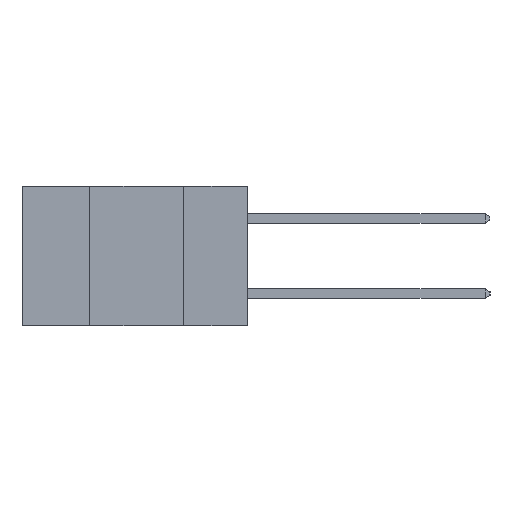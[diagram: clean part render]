
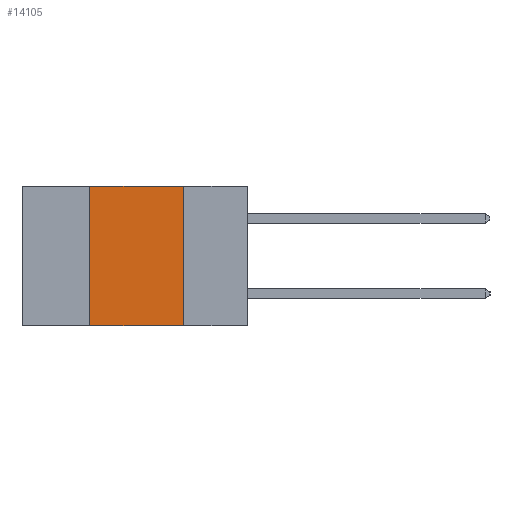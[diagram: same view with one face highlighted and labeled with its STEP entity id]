
A CAD part, left-side view. The second image highlights one B-rep face of the part: STEP entity #14105.
In plain terms, the highlighted planar face has unit normal (-1, 0, 0).
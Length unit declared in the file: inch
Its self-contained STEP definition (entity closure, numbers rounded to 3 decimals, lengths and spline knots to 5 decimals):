
#22 = ORIENTED_EDGE ( 'NONE', *, *, #12475, .F. ) ;
#81 = DIRECTION ( 'NONE',  ( 0., -1., 0. ) ) ;
#1316 = VERTEX_POINT ( 'NONE', #8746 ) ;
#1593 = VECTOR ( 'NONE', #3439, 39.37008 ) ;
#1913 = EDGE_CURVE ( 'NONE', #6254, #7002, #3189, .T. ) ;
#1920 = VERTEX_POINT ( 'NONE', #11821 ) ;
#2211 = CARTESIAN_POINT ( 'NONE',  ( 0., 0.42, -0.37 ) ) ;
#2254 = DIRECTION ( 'NONE',  ( 0., 0., 1. ) ) ;
#3166 = ORIENTED_EDGE ( 'NONE', *, *, #1913, .F. ) ;
#3189 = LINE ( 'NONE', #5983, #9202 ) ;
#3439 = DIRECTION ( 'NONE',  ( 0., 0., -1. ) ) ;
#3627 = LINE ( 'NONE', #2211, #10006 ) ;
#4427 = CARTESIAN_POINT ( 'NONE',  ( 0., 0.17, -0.37 ) ) ;
#4511 = CARTESIAN_POINT ( 'NONE',  ( 0., 0.42, 0. ) ) ;
#5983 = CARTESIAN_POINT ( 'NONE',  ( 0., 0.6, 0. ) ) ;
#6254 = VERTEX_POINT ( 'NONE', #4511 ) ;
#6740 = CARTESIAN_POINT ( 'NONE',  ( 0., 0.17, 0. ) ) ;
#6757 = EDGE_CURVE ( 'NONE', #1920, #6254, #3627, .T. ) ;
#6924 = DIRECTION ( 'NONE',  ( 0., 0., -1. ) ) ;
#7002 = VERTEX_POINT ( 'NONE', #6740 ) ;
#7289 = VECTOR ( 'NONE', #81, 39.37008 ) ;
#7996 = LINE ( 'NONE', #4427, #1593 ) ;
#8746 = CARTESIAN_POINT ( 'NONE',  ( 0., 0.17, -0.37 ) ) ;
#8836 = DIRECTION ( 'NONE',  ( 0., -1., 0. ) ) ;
#9202 = VECTOR ( 'NONE', #8836, 39.37008 ) ;
#9536 = ORIENTED_EDGE ( 'NONE', *, *, #6757, .F. ) ;
#10006 = VECTOR ( 'NONE', #2254, 39.37008 ) ;
#10420 = LINE ( 'NONE', #12936, #7289 ) ;
#10441 = PLANE ( 'NONE',  #10904 ) ;
#10904 = AXIS2_PLACEMENT_3D ( 'NONE', #12666, #13755, #6924 ) ;
#11821 = CARTESIAN_POINT ( 'NONE',  ( 0., 0.42, -0.37 ) ) ;
#12475 = EDGE_CURVE ( 'NONE', #7002, #1316, #7996, .T. ) ;
#12519 = ORIENTED_EDGE ( 'NONE', *, *, #12937, .T. ) ;
#12666 = CARTESIAN_POINT ( 'NONE',  ( 0., 0.6, 0. ) ) ;
#12790 = EDGE_LOOP ( 'NONE', ( #22, #3166, #9536, #12519 ) ) ;
#12936 = CARTESIAN_POINT ( 'NONE',  ( 0., 0.6, -0.37 ) ) ;
#12937 = EDGE_CURVE ( 'NONE', #1920, #1316, #10420, .T. ) ;
#13755 = DIRECTION ( 'NONE',  ( 1., 0., 0. ) ) ;
#14105 = ADVANCED_FACE ( 'NONE', ( #14877 ), #10441, .F. ) ;
#14877 = FACE_OUTER_BOUND ( 'NONE', #12790, .T. ) ;
